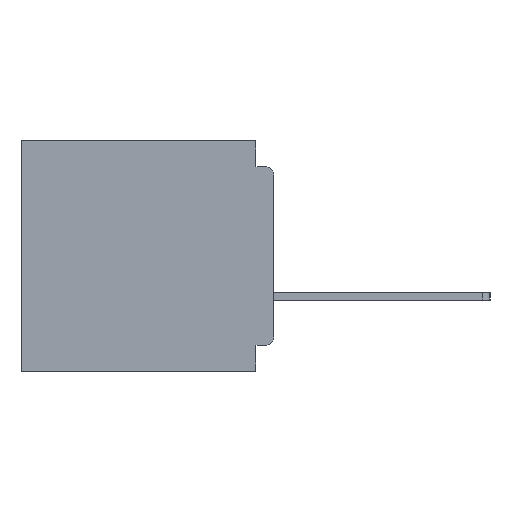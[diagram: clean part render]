
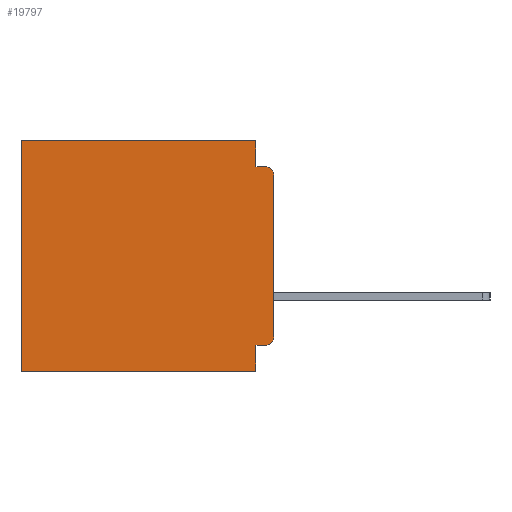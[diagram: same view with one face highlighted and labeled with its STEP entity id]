
A CAD part, left-side view. The second image highlights one B-rep face of the part: STEP entity #19797.
In plain terms, the highlighted planar face has unit normal (-1, 0, 0).
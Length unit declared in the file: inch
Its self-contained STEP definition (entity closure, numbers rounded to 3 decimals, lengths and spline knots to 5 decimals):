
#204 = CARTESIAN_POINT ( 'NONE',  ( 0.3, 0.031, -0.4 ) ) ;
#1154 = CARTESIAN_POINT ( 'NONE',  ( 0.3, 0., -0.34 ) ) ;
#1630 = PLANE ( 'NONE',  #43378 ) ;
#2743 = DIRECTION ( 'NONE',  ( 0., -1., 0. ) ) ;
#2914 = VERTEX_POINT ( 'NONE', #36855 ) ;
#3016 = ORIENTED_EDGE ( 'NONE', *, *, #35074, .T. ) ;
#3351 = CIRCLE ( 'NONE', #55890, 0.015 ) ;
#5212 = EDGE_CURVE ( 'NONE', #21621, #11869, #44126, .T. ) ;
#6082 = CARTESIAN_POINT ( 'NONE',  ( 0.3, 0., -0.06 ) ) ;
#6774 = EDGE_CURVE ( 'NONE', #11869, #20975, #46530, .T. ) ;
#7401 = VERTEX_POINT ( 'NONE', #8168 ) ;
#8168 = CARTESIAN_POINT ( 'NONE',  ( 0.3, 0.015, -0.355 ) ) ;
#9143 = VECTOR ( 'NONE', #48915, 39.37008 ) ;
#9505 = VERTEX_POINT ( 'NONE', #15576 ) ;
#9565 = CARTESIAN_POINT ( 'NONE',  ( 0.3, 0., -0.4 ) ) ;
#9740 = VECTOR ( 'NONE', #55668, 39.37008 ) ;
#10208 = ORIENTED_EDGE ( 'NONE', *, *, #56101, .F. ) ;
#10281 = VECTOR ( 'NONE', #2743, 39.37008 ) ;
#10638 = CARTESIAN_POINT ( 'NONE',  ( 0.3, 0.015, -0.06 ) ) ;
#11329 = EDGE_CURVE ( 'NONE', #43847, #20975, #11565, .T. ) ;
#11427 = CARTESIAN_POINT ( 'NONE',  ( 0.3, 0.437, -0.4 ) ) ;
#11565 = LINE ( 'NONE', #24315, #59810 ) ;
#11869 = VERTEX_POINT ( 'NONE', #204 ) ;
#12963 = EDGE_CURVE ( 'NONE', #30726, #16300, #30003, .T. ) ;
#14062 = DIRECTION ( 'NONE',  ( -1., 0., 0. ) ) ;
#14600 = ORIENTED_EDGE ( 'NONE', *, *, #58244, .F. ) ;
#15409 = DIRECTION ( 'NONE',  ( 0., 0., -1. ) ) ;
#15576 = CARTESIAN_POINT ( 'NONE',  ( 0.3, 0.015, -0.045 ) ) ;
#15892 = DIRECTION ( 'NONE',  ( 1., 0., 0. ) ) ;
#16300 = VERTEX_POINT ( 'NONE', #1154 ) ;
#17138 = ORIENTED_EDGE ( 'NONE', *, *, #6774, .F. ) ;
#19797 = ADVANCED_FACE ( 'NONE', ( #54067 ), #1630, .F. ) ;
#20288 = ORIENTED_EDGE ( 'NONE', *, *, #43148, .T. ) ;
#20975 = VERTEX_POINT ( 'NONE', #11427 ) ;
#21471 = EDGE_LOOP ( 'NONE', ( #28766, #3016, #14600, #10208, #26360, #41165, #17138, #55058, #50107, #20288 ) ) ;
#21621 = VERTEX_POINT ( 'NONE', #54600 ) ;
#22259 = LINE ( 'NONE', #46316, #9740 ) ;
#23501 = DIRECTION ( 'NONE',  ( 0., 1., 0. ) ) ;
#24315 = CARTESIAN_POINT ( 'NONE',  ( 0.3, 0.437, -0.4 ) ) ;
#26212 = VECTOR ( 'NONE', #60597, 39.37008 ) ;
#26360 = ORIENTED_EDGE ( 'NONE', *, *, #38712, .T. ) ;
#27753 = EDGE_CURVE ( 'NONE', #7401, #21621, #49640, .T. ) ;
#27994 = CARTESIAN_POINT ( 'NONE',  ( 0.3, 0., -0.355 ) ) ;
#28766 = ORIENTED_EDGE ( 'NONE', *, *, #12963, .F. ) ;
#30003 = LINE ( 'NONE', #9565, #56327 ) ;
#30726 = VERTEX_POINT ( 'NONE', #6082 ) ;
#35074 = EDGE_CURVE ( 'NONE', #30726, #9505, #3351, .T. ) ;
#35625 = CARTESIAN_POINT ( 'NONE',  ( 0.3, 0., -0.045 ) ) ;
#36715 = AXIS2_PLACEMENT_3D ( 'NONE', #42090, #14062, #46783 ) ;
#36732 = LINE ( 'NONE', #35625, #10281 ) ;
#36855 = CARTESIAN_POINT ( 'NONE',  ( 0.3, 0.031, -0.045 ) ) ;
#37149 = DIRECTION ( 'NONE',  ( 0., 0., -1. ) ) ;
#37201 = CARTESIAN_POINT ( 'NONE',  ( 0.3, 0.031, -0.4 ) ) ;
#38712 = EDGE_CURVE ( 'NONE', #45637, #43847, #59458, .T. ) ;
#41165 = ORIENTED_EDGE ( 'NONE', *, *, #11329, .T. ) ;
#42090 = CARTESIAN_POINT ( 'NONE',  ( 0.3, 0.015, -0.34 ) ) ;
#42368 = DIRECTION ( 'NONE',  ( 0., 0., -1. ) ) ;
#43148 = EDGE_CURVE ( 'NONE', #7401, #16300, #43370, .T. ) ;
#43170 = DIRECTION ( 'NONE',  ( 0., 0., -1. ) ) ;
#43370 = CIRCLE ( 'NONE', #36715, 0.015 ) ;
#43378 = AXIS2_PLACEMENT_3D ( 'NONE', #57731, #15892, #48595 ) ;
#43425 = DIRECTION ( 'NONE',  ( -1., 0., 0. ) ) ;
#43847 = VERTEX_POINT ( 'NONE', #51777 ) ;
#44126 = LINE ( 'NONE', #37201, #45628 ) ;
#45628 = VECTOR ( 'NONE', #37149, 39.37008 ) ;
#45637 = VERTEX_POINT ( 'NONE', #46014 ) ;
#46014 = CARTESIAN_POINT ( 'NONE',  ( 0.3, 0.031, 0. ) ) ;
#46316 = CARTESIAN_POINT ( 'NONE',  ( 0.3, 0.031, 0. ) ) ;
#46530 = LINE ( 'NONE', #50757, #9143 ) ;
#46783 = DIRECTION ( 'NONE',  ( 0., 0., -1. ) ) ;
#47126 = VECTOR ( 'NONE', #23501, 39.37008 ) ;
#48595 = DIRECTION ( 'NONE',  ( 0., 0., -1. ) ) ;
#48915 = DIRECTION ( 'NONE',  ( 0., 1., 0. ) ) ;
#49640 = LINE ( 'NONE', #27994, #26212 ) ;
#50107 = ORIENTED_EDGE ( 'NONE', *, *, #27753, .F. ) ;
#50757 = CARTESIAN_POINT ( 'NONE',  ( 0.3, 0., -0.4 ) ) ;
#51311 = CARTESIAN_POINT ( 'NONE',  ( 0.3, 0., 0. ) ) ;
#51777 = CARTESIAN_POINT ( 'NONE',  ( 0.3, 0.437, 0. ) ) ;
#54067 = FACE_OUTER_BOUND ( 'NONE', #21471, .T. ) ;
#54600 = CARTESIAN_POINT ( 'NONE',  ( 0.3, 0.031, -0.355 ) ) ;
#55058 = ORIENTED_EDGE ( 'NONE', *, *, #5212, .F. ) ;
#55668 = DIRECTION ( 'NONE',  ( 0., 0., -1. ) ) ;
#55890 = AXIS2_PLACEMENT_3D ( 'NONE', #10638, #43425, #15409 ) ;
#56101 = EDGE_CURVE ( 'NONE', #45637, #2914, #22259, .T. ) ;
#56327 = VECTOR ( 'NONE', #42368, 39.37008 ) ;
#57731 = CARTESIAN_POINT ( 'NONE',  ( 0.3, 0., -0.4 ) ) ;
#58244 = EDGE_CURVE ( 'NONE', #2914, #9505, #36732, .T. ) ;
#59458 = LINE ( 'NONE', #51311, #47126 ) ;
#59810 = VECTOR ( 'NONE', #43170, 39.37008 ) ;
#60597 = DIRECTION ( 'NONE',  ( 0., 1., 0. ) ) ;
